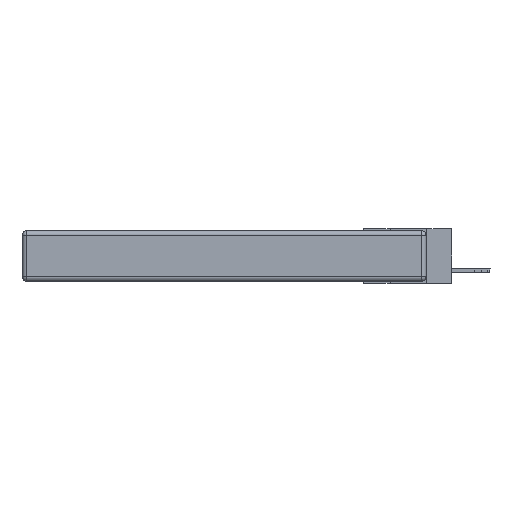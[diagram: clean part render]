
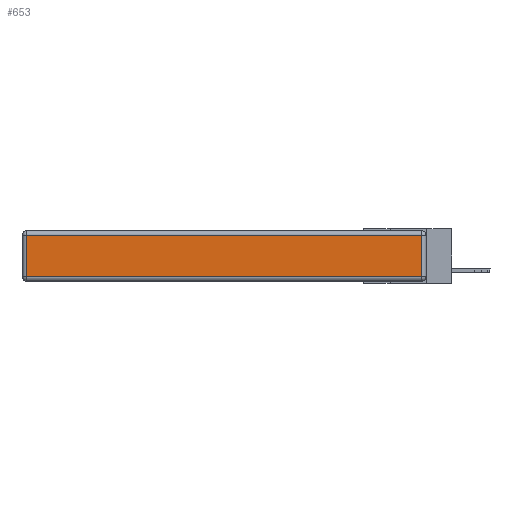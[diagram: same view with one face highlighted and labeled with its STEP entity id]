
A CAD part, left-side view. The second image highlights one B-rep face of the part: STEP entity #653.
In plain terms, the highlighted planar face has unit normal (-1, 0, 0).
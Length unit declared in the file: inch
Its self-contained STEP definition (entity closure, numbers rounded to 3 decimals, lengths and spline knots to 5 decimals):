
#188 = ORIENTED_EDGE ( 'NONE', *, *, #5144, .T. ) ;
#360 = EDGE_LOOP ( 'NONE', ( #3748, #10366, #13486, #188 ) ) ;
#439 = EDGE_CURVE ( 'NONE', #8534, #5061, #7974, .T. ) ;
#484 = DIRECTION ( 'NONE',  ( 0., 1., 0. ) ) ;
#653 = ADVANCED_FACE ( 'NONE', ( #7532 ), #17459, .T. ) ;
#3147 = CARTESIAN_POINT ( 'NONE',  ( 0., 2.75, -0.03 ) ) ;
#3507 = LINE ( 'NONE', #3147, #16148 ) ;
#3536 = CARTESIAN_POINT ( 'NONE',  ( 0., 2.72, -0.313 ) ) ;
#3748 = ORIENTED_EDGE ( 'NONE', *, *, #11384, .T. ) ;
#5061 = VERTEX_POINT ( 'NONE', #12010 ) ;
#5144 = EDGE_CURVE ( 'NONE', #17155, #12025, #10330, .T. ) ;
#5290 = DIRECTION ( 'NONE',  ( 0., 0., -1. ) ) ;
#5847 = VECTOR ( 'NONE', #6414, 39.37008 ) ;
#6170 = CARTESIAN_POINT ( 'NONE',  ( 0., 0.03, -0.343 ) ) ;
#6414 = DIRECTION ( 'NONE',  ( 0., 0., 1. ) ) ;
#6536 = CARTESIAN_POINT ( 'NONE',  ( 0., 2.72, -0.343 ) ) ;
#6796 = AXIS2_PLACEMENT_3D ( 'NONE', #14808, #14925, #16157 ) ;
#7532 = FACE_OUTER_BOUND ( 'NONE', #360, .T. ) ;
#7974 = LINE ( 'NONE', #6170, #5847 ) ;
#8534 = VERTEX_POINT ( 'NONE', #9224 ) ;
#9224 = CARTESIAN_POINT ( 'NONE',  ( 0., 0.03, -0.313 ) ) ;
#10033 = CARTESIAN_POINT ( 'NONE',  ( 0., 0., -0.313 ) ) ;
#10215 = DIRECTION ( 'NONE',  ( 0., -1., 0. ) ) ;
#10330 = LINE ( 'NONE', #6536, #17062 ) ;
#10366 = ORIENTED_EDGE ( 'NONE', *, *, #439, .T. ) ;
#10431 = LINE ( 'NONE', #10033, #15069 ) ;
#11384 = EDGE_CURVE ( 'NONE', #12025, #8534, #10431, .T. ) ;
#12010 = CARTESIAN_POINT ( 'NONE',  ( 0., 0.03, -0.03 ) ) ;
#12025 = VERTEX_POINT ( 'NONE', #3536 ) ;
#13486 = ORIENTED_EDGE ( 'NONE', *, *, #17478, .T. ) ;
#14808 = CARTESIAN_POINT ( 'NONE',  ( 0., 0., -0.343 ) ) ;
#14821 = CARTESIAN_POINT ( 'NONE',  ( 0., 2.72, -0.03 ) ) ;
#14925 = DIRECTION ( 'NONE',  ( -1., 0., 0. ) ) ;
#15069 = VECTOR ( 'NONE', #10215, 39.37008 ) ;
#16148 = VECTOR ( 'NONE', #484, 39.37008 ) ;
#16157 = DIRECTION ( 'NONE',  ( 0., 0., 1. ) ) ;
#17062 = VECTOR ( 'NONE', #5290, 39.37008 ) ;
#17155 = VERTEX_POINT ( 'NONE', #14821 ) ;
#17459 = PLANE ( 'NONE',  #6796 ) ;
#17478 = EDGE_CURVE ( 'NONE', #5061, #17155, #3507, .T. ) ;
